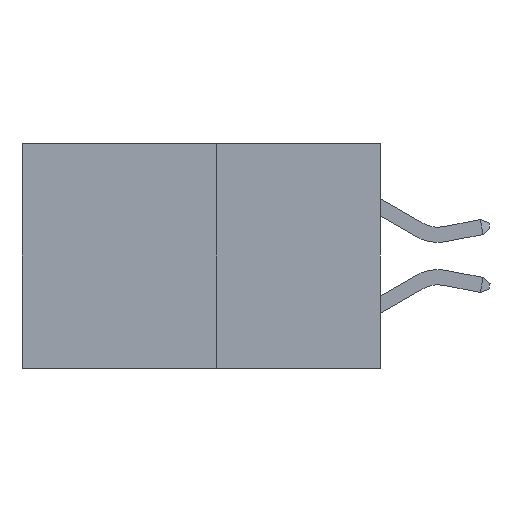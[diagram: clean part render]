
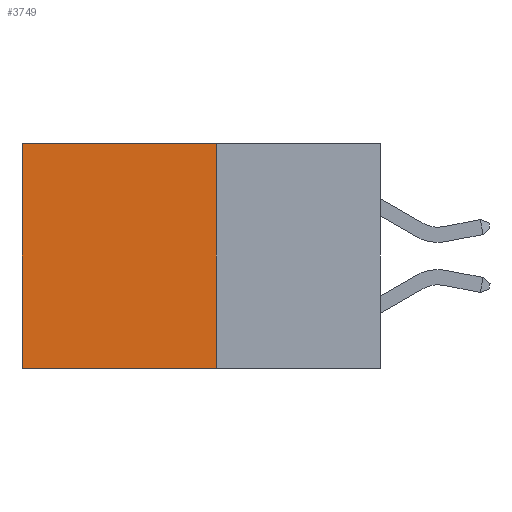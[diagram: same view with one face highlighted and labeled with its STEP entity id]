
A CAD part, left-side view. The second image highlights one B-rep face of the part: STEP entity #3749.
In plain terms, the highlighted planar face has unit normal (-1, 0, 0).
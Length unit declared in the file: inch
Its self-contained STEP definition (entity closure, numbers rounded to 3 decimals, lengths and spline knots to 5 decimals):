
#19 = PLANE ( 'NONE',  #3315 ) ;
#274 = DIRECTION ( 'NONE',  ( 0., 0., -1. ) ) ;
#617 = CARTESIAN_POINT ( 'NONE',  ( 0.277, 0.59, -0.37 ) ) ;
#982 = ORIENTED_EDGE ( 'NONE', *, *, #8758, .T. ) ;
#996 = LINE ( 'NONE', #3868, #7324 ) ;
#1419 = CARTESIAN_POINT ( 'NONE',  ( 0.277, 0.27, 0. ) ) ;
#1672 = VERTEX_POINT ( 'NONE', #11786 ) ;
#1994 = DIRECTION ( 'NONE',  ( 0., 0., -1. ) ) ;
#2237 = EDGE_LOOP ( 'NONE', ( #15226, #11036, #11221, #982 ) ) ;
#3179 = CARTESIAN_POINT ( 'NONE',  ( 0.277, 0.59, -0.37 ) ) ;
#3242 = LINE ( 'NONE', #3423, #12708 ) ;
#3315 = AXIS2_PLACEMENT_3D ( 'NONE', #5431, #13960, #274 ) ;
#3423 = CARTESIAN_POINT ( 'NONE',  ( 0.277, 0.27, -0.37 ) ) ;
#3749 = ADVANCED_FACE ( 'NONE', ( #14109 ), #19, .F. ) ;
#3868 = CARTESIAN_POINT ( 'NONE',  ( 0.277, 0.27, 0. ) ) ;
#4635 = VECTOR ( 'NONE', #8213, 39.37008 ) ;
#4716 = LINE ( 'NONE', #3179, #10698 ) ;
#5431 = CARTESIAN_POINT ( 'NONE',  ( 0.277, 0.27, -0.37 ) ) ;
#5490 = CARTESIAN_POINT ( 'NONE',  ( 0.277, 0.59, 0. ) ) ;
#7197 = VERTEX_POINT ( 'NONE', #1419 ) ;
#7324 = VECTOR ( 'NONE', #13352, 39.37008 ) ;
#7811 = LINE ( 'NONE', #10588, #4635 ) ;
#8213 = DIRECTION ( 'NONE',  ( 0., 0., -1. ) ) ;
#8456 = EDGE_CURVE ( 'NONE', #11461, #13933, #4716, .T. ) ;
#8758 = EDGE_CURVE ( 'NONE', #7197, #11461, #996, .T. ) ;
#10588 = CARTESIAN_POINT ( 'NONE',  ( 0.277, 0.27, -0.37 ) ) ;
#10698 = VECTOR ( 'NONE', #1994, 39.37008 ) ;
#11036 = ORIENTED_EDGE ( 'NONE', *, *, #14609, .F. ) ;
#11221 = ORIENTED_EDGE ( 'NONE', *, *, #11652, .F. ) ;
#11461 = VERTEX_POINT ( 'NONE', #5490 ) ;
#11652 = EDGE_CURVE ( 'NONE', #7197, #1672, #7811, .T. ) ;
#11726 = DIRECTION ( 'NONE',  ( 0., 1., 0. ) ) ;
#11786 = CARTESIAN_POINT ( 'NONE',  ( 0.277, 0.27, -0.37 ) ) ;
#12708 = VECTOR ( 'NONE', #11726, 39.37008 ) ;
#13352 = DIRECTION ( 'NONE',  ( 0., 1., 0. ) ) ;
#13933 = VERTEX_POINT ( 'NONE', #617 ) ;
#13960 = DIRECTION ( 'NONE',  ( 1., 0., 0. ) ) ;
#14109 = FACE_OUTER_BOUND ( 'NONE', #2237, .T. ) ;
#14609 = EDGE_CURVE ( 'NONE', #1672, #13933, #3242, .T. ) ;
#15226 = ORIENTED_EDGE ( 'NONE', *, *, #8456, .T. ) ;
